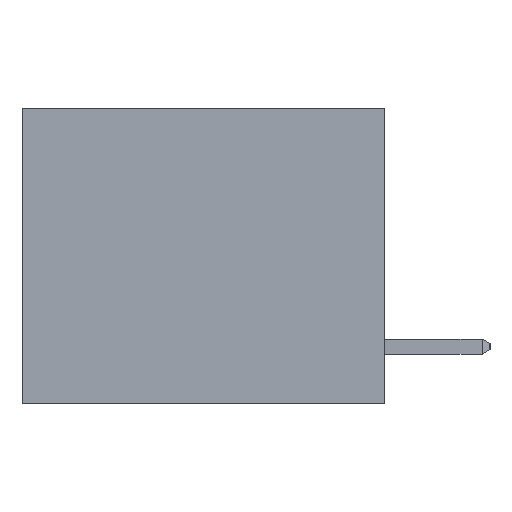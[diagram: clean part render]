
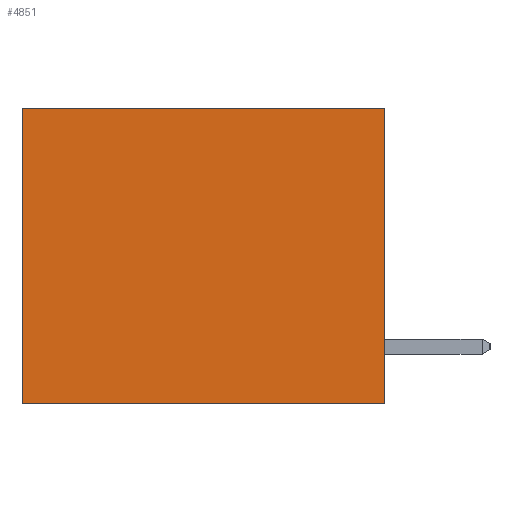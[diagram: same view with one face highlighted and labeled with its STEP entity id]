
A CAD part, left-side view. The second image highlights one B-rep face of the part: STEP entity #4851.
In plain terms, the highlighted planar face has unit normal (-1, 0, 0).
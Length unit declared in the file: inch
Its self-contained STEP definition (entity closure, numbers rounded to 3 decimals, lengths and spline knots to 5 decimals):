
#668 = FACE_OUTER_BOUND ( 'NONE', #2045, .T. ) ;
#815 = DIRECTION ( 'NONE',  ( 0., 1., 0. ) ) ;
#1568 = CARTESIAN_POINT ( 'NONE',  ( 0.3165, 0.6, -0.49 ) ) ;
#2045 = EDGE_LOOP ( 'NONE', ( #7711, #9928, #14498, #5778 ) ) ;
#2246 = CARTESIAN_POINT ( 'NONE',  ( 0.3165, 0., -0.49 ) ) ;
#2380 = VECTOR ( 'NONE', #815, 39.37008 ) ;
#2588 = CARTESIAN_POINT ( 'NONE',  ( 0.3165, 0., 0. ) ) ;
#3166 = VERTEX_POINT ( 'NONE', #2588 ) ;
#3996 = EDGE_CURVE ( 'NONE', #3166, #6019, #6271, .T. ) ;
#4468 = CARTESIAN_POINT ( 'NONE',  ( 0.3165, 0., -0.49 ) ) ;
#4851 = ADVANCED_FACE ( 'NONE', ( #668 ), #8667, .F. ) ;
#5037 = VERTEX_POINT ( 'NONE', #17178 ) ;
#5152 = VECTOR ( 'NONE', #14549, 39.37008 ) ;
#5778 = ORIENTED_EDGE ( 'NONE', *, *, #7499, .T. ) ;
#6019 = VERTEX_POINT ( 'NONE', #19256 ) ;
#6271 = LINE ( 'NONE', #6439, #18818 ) ;
#6439 = CARTESIAN_POINT ( 'NONE',  ( 0.3165, 0., -0.49 ) ) ;
#7037 = LINE ( 'NONE', #2246, #5152 ) ;
#7434 = CARTESIAN_POINT ( 'NONE',  ( 0.3165, 0.6, 0. ) ) ;
#7499 = EDGE_CURVE ( 'NONE', #3166, #13499, #23386, .T. ) ;
#7711 = ORIENTED_EDGE ( 'NONE', *, *, #21174, .T. ) ;
#8655 = EDGE_CURVE ( 'NONE', #6019, #5037, #7037, .T. ) ;
#8667 = PLANE ( 'NONE',  #11804 ) ;
#9320 = VECTOR ( 'NONE', #11730, 39.37008 ) ;
#9928 = ORIENTED_EDGE ( 'NONE', *, *, #8655, .F. ) ;
#10628 = DIRECTION ( 'NONE',  ( 0., 0., -1. ) ) ;
#11730 = DIRECTION ( 'NONE',  ( 0., 0., -1. ) ) ;
#11804 = AXIS2_PLACEMENT_3D ( 'NONE', #4468, #20582, #10628 ) ;
#13499 = VERTEX_POINT ( 'NONE', #7434 ) ;
#13719 = LINE ( 'NONE', #1568, #9320 ) ;
#14498 = ORIENTED_EDGE ( 'NONE', *, *, #3996, .F. ) ;
#14549 = DIRECTION ( 'NONE',  ( 0., 1., 0. ) ) ;
#17178 = CARTESIAN_POINT ( 'NONE',  ( 0.3165, 0.6, -0.49 ) ) ;
#18818 = VECTOR ( 'NONE', #20456, 39.37008 ) ;
#19256 = CARTESIAN_POINT ( 'NONE',  ( 0.3165, 0., -0.49 ) ) ;
#20456 = DIRECTION ( 'NONE',  ( 0., 0., -1. ) ) ;
#20582 = DIRECTION ( 'NONE',  ( 1., 0., 0. ) ) ;
#21174 = EDGE_CURVE ( 'NONE', #13499, #5037, #13719, .T. ) ;
#21451 = CARTESIAN_POINT ( 'NONE',  ( 0.3165, 0., 0. ) ) ;
#23386 = LINE ( 'NONE', #21451, #2380 ) ;
